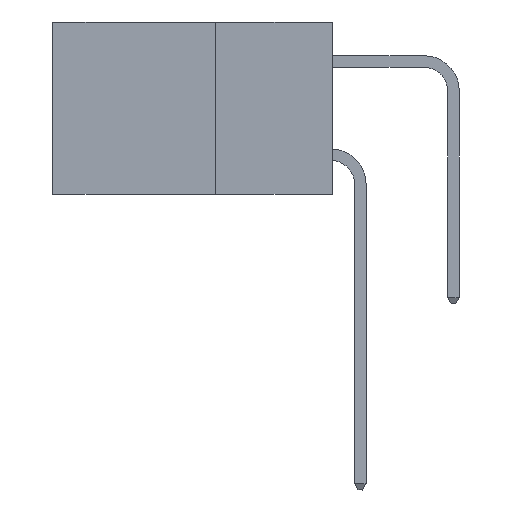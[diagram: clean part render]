
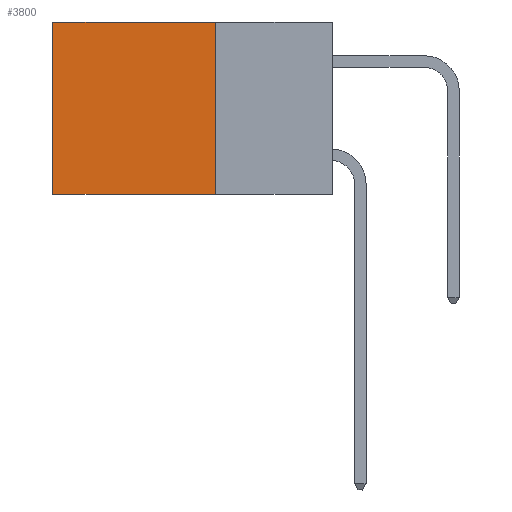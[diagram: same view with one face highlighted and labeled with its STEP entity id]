
A CAD part, left-side view. The second image highlights one B-rep face of the part: STEP entity #3800.
In plain terms, the highlighted planar face has unit normal (-1, 0, 0).
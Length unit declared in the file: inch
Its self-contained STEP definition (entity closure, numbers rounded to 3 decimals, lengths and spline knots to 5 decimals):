
#1071 = EDGE_CURVE ( 'NONE', #11617, #8645, #11800, .T. ) ;
#2204 = ORIENTED_EDGE ( 'NONE', *, *, #7752, .F. ) ;
#2566 = VECTOR ( 'NONE', #2646, 39.37008 ) ;
#2646 = DIRECTION ( 'NONE',  ( 0., 1., 0. ) ) ;
#3467 = CARTESIAN_POINT ( 'NONE',  ( 0.2615, 0.25, -0.37 ) ) ;
#3800 = ADVANCED_FACE ( 'NONE', ( #17997 ), #6873, .F. ) ;
#5024 = CARTESIAN_POINT ( 'NONE',  ( 0.2615, 0.25, 0. ) ) ;
#5895 = VERTEX_POINT ( 'NONE', #15265 ) ;
#6873 = PLANE ( 'NONE',  #16980 ) ;
#7752 = EDGE_CURVE ( 'NONE', #20037, #11617, #8181, .T. ) ;
#7930 = CARTESIAN_POINT ( 'NONE',  ( 0.2615, 0.25, -0.37 ) ) ;
#8181 = LINE ( 'NONE', #7930, #19282 ) ;
#8248 = CARTESIAN_POINT ( 'NONE',  ( 0.2615, 0.25, -0.37 ) ) ;
#8645 = VERTEX_POINT ( 'NONE', #11146 ) ;
#9951 = CARTESIAN_POINT ( 'NONE',  ( 0.2615, 0.25, -0.37 ) ) ;
#10091 = CARTESIAN_POINT ( 'NONE',  ( 0.2615, 0.25, 0. ) ) ;
#10115 = CARTESIAN_POINT ( 'NONE',  ( 0.2615, 0.6, -0.37 ) ) ;
#11146 = CARTESIAN_POINT ( 'NONE',  ( 0.2615, 0.6, -0.37 ) ) ;
#11617 = VERTEX_POINT ( 'NONE', #3467 ) ;
#11800 = LINE ( 'NONE', #9951, #2566 ) ;
#12272 = VECTOR ( 'NONE', #17638, 39.37008 ) ;
#12395 = ORIENTED_EDGE ( 'NONE', *, *, #23197, .T. ) ;
#12579 = DIRECTION ( 'NONE',  ( 0., 1., 0. ) ) ;
#13816 = LINE ( 'NONE', #10115, #12272 ) ;
#13940 = DIRECTION ( 'NONE',  ( 0., 0., -1. ) ) ;
#14099 = EDGE_CURVE ( 'NONE', #5895, #8645, #13816, .T. ) ;
#15265 = CARTESIAN_POINT ( 'NONE',  ( 0.2615, 0.6, 0. ) ) ;
#15693 = ORIENTED_EDGE ( 'NONE', *, *, #14099, .T. ) ;
#16649 = VECTOR ( 'NONE', #12579, 39.37008 ) ;
#16980 = AXIS2_PLACEMENT_3D ( 'NONE', #8248, #23307, #13940 ) ;
#17638 = DIRECTION ( 'NONE',  ( 0., 0., -1. ) ) ;
#17997 = FACE_OUTER_BOUND ( 'NONE', #23832, .T. ) ;
#19282 = VECTOR ( 'NONE', #19399, 39.37008 ) ;
#19399 = DIRECTION ( 'NONE',  ( 0., 0., -1. ) ) ;
#20037 = VERTEX_POINT ( 'NONE', #10091 ) ;
#21784 = ORIENTED_EDGE ( 'NONE', *, *, #1071, .F. ) ;
#21946 = LINE ( 'NONE', #5024, #16649 ) ;
#23197 = EDGE_CURVE ( 'NONE', #20037, #5895, #21946, .T. ) ;
#23307 = DIRECTION ( 'NONE',  ( 1., 0., 0. ) ) ;
#23832 = EDGE_LOOP ( 'NONE', ( #15693, #21784, #2204, #12395 ) ) ;
